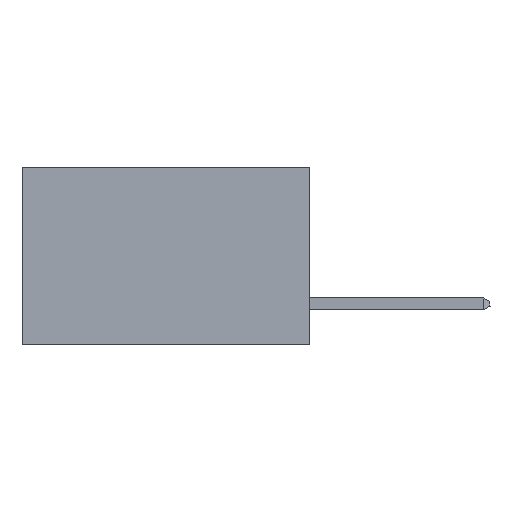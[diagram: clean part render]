
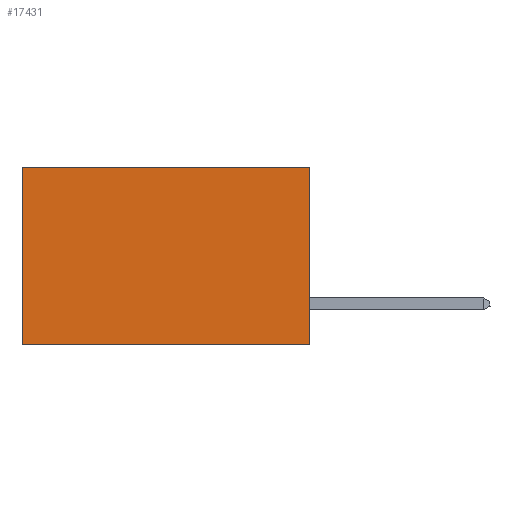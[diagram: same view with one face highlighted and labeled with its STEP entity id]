
A CAD part, left-side view. The second image highlights one B-rep face of the part: STEP entity #17431.
In plain terms, the highlighted planar face has unit normal (-1, 0, 0).
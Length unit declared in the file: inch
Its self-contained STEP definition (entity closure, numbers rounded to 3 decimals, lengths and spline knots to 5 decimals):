
#261 = EDGE_CURVE ( 'NONE', #39543, #42862, #40807, .T. ) ;
#4017 = VERTEX_POINT ( 'NONE', #12187 ) ;
#5389 = EDGE_CURVE ( 'NONE', #4017, #42862, #36642, .T. ) ;
#6105 = CARTESIAN_POINT ( 'NONE',  ( 0.2875, 0., 0. ) ) ;
#6525 = VECTOR ( 'NONE', #11245, 39.37008 ) ;
#6706 = DIRECTION ( 'NONE',  ( 0., 1., 0. ) ) ;
#7267 = CARTESIAN_POINT ( 'NONE',  ( 0.2875, 0., 0. ) ) ;
#7484 = ORIENTED_EDGE ( 'NONE', *, *, #15044, .F. ) ;
#10948 = DIRECTION ( 'NONE',  ( 0., 0., -1. ) ) ;
#11245 = DIRECTION ( 'NONE',  ( 0., 0., -1. ) ) ;
#12187 = CARTESIAN_POINT ( 'NONE',  ( 0.2875, 0.6, 0. ) ) ;
#13767 = EDGE_LOOP ( 'NONE', ( #34534, #38247, #7484, #34537 ) ) ;
#15044 = EDGE_CURVE ( 'NONE', #36399, #39543, #44846, .T. ) ;
#17268 = VECTOR ( 'NONE', #24990, 39.37008 ) ;
#17431 = ADVANCED_FACE ( 'NONE', ( #41218 ), #25850, .F. ) ;
#24990 = DIRECTION ( 'NONE',  ( 0., 0., -1. ) ) ;
#25850 = PLANE ( 'NONE',  #27802 ) ;
#26003 = DIRECTION ( 'NONE',  ( 1., 0., 0. ) ) ;
#27802 = AXIS2_PLACEMENT_3D ( 'NONE', #7267, #26003, #10948 ) ;
#29830 = CARTESIAN_POINT ( 'NONE',  ( 0.2875, 0., 0. ) ) ;
#30536 = VECTOR ( 'NONE', #6706, 39.37008 ) ;
#32019 = EDGE_CURVE ( 'NONE', #36399, #4017, #32273, .T. ) ;
#32159 = CARTESIAN_POINT ( 'NONE',  ( 0.2875, 0., 0. ) ) ;
#32273 = LINE ( 'NONE', #32159, #30536 ) ;
#34534 = ORIENTED_EDGE ( 'NONE', *, *, #5389, .T. ) ;
#34537 = ORIENTED_EDGE ( 'NONE', *, *, #32019, .T. ) ;
#35650 = CARTESIAN_POINT ( 'NONE',  ( 0.2875, 0.6, 0. ) ) ;
#36399 = VERTEX_POINT ( 'NONE', #6105 ) ;
#36642 = LINE ( 'NONE', #35650, #17268 ) ;
#36859 = CARTESIAN_POINT ( 'NONE',  ( 0.2875, 0., -0.37 ) ) ;
#37015 = DIRECTION ( 'NONE',  ( 0., 1., 0. ) ) ;
#38247 = ORIENTED_EDGE ( 'NONE', *, *, #261, .F. ) ;
#38571 = CARTESIAN_POINT ( 'NONE',  ( 0.2875, 0.6, -0.37 ) ) ;
#39543 = VERTEX_POINT ( 'NONE', #39909 ) ;
#39909 = CARTESIAN_POINT ( 'NONE',  ( 0.2875, 0., -0.37 ) ) ;
#40235 = VECTOR ( 'NONE', #37015, 39.37008 ) ;
#40807 = LINE ( 'NONE', #36859, #40235 ) ;
#41218 = FACE_OUTER_BOUND ( 'NONE', #13767, .T. ) ;
#42862 = VERTEX_POINT ( 'NONE', #38571 ) ;
#44846 = LINE ( 'NONE', #29830, #6525 ) ;
